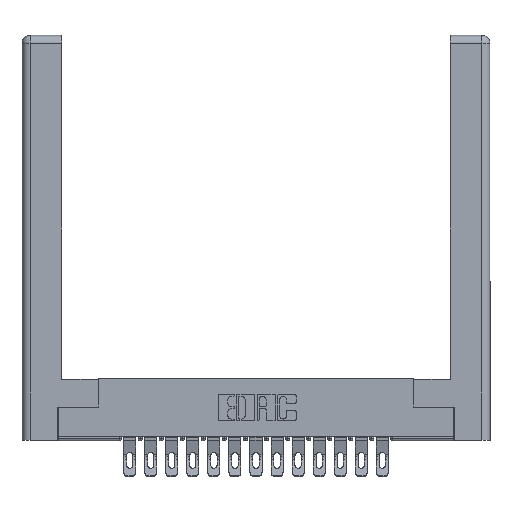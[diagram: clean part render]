
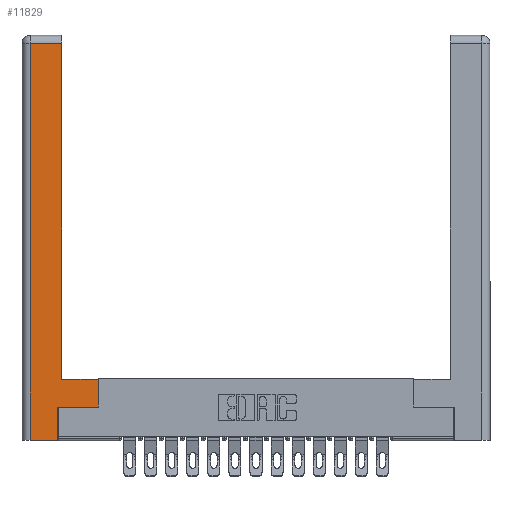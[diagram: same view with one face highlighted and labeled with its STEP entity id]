
A CAD part, top view. The second image highlights one B-rep face of the part: STEP entity #11829.
In plain terms, the highlighted planar face has unit normal (0, 0, 1).
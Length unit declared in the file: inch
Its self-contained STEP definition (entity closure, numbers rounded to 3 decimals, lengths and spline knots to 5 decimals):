
#189 = CARTESIAN_POINT ( 'NONE',  ( 0.265, 0., 0. ) ) ;
#281 = CARTESIAN_POINT ( 'NONE',  ( 0.0615, 2.94, 0. ) ) ;
#295 = PLANE ( 'NONE',  #5100 ) ;
#472 = EDGE_CURVE ( 'NONE', #750, #2969, #9812, .T. ) ;
#750 = VERTEX_POINT ( 'NONE', #14348 ) ;
#1645 = EDGE_CURVE ( 'NONE', #14276, #2510, #8783, .T. ) ;
#2114 = EDGE_CURVE ( 'NONE', #15263, #13758, #15325, .T. ) ;
#2134 = CARTESIAN_POINT ( 'NONE',  ( 0., 0., 0. ) ) ;
#2287 = DIRECTION ( 'NONE',  ( 0., 1., 0. ) ) ;
#2510 = VERTEX_POINT ( 'NONE', #15533 ) ;
#2518 = ORIENTED_EDGE ( 'NONE', *, *, #9903, .T. ) ;
#2969 = VERTEX_POINT ( 'NONE', #12565 ) ;
#3335 = CARTESIAN_POINT ( 'NONE',  ( 0.265, 0., 0. ) ) ;
#3421 = VERTEX_POINT ( 'NONE', #3335 ) ;
#4067 = VECTOR ( 'NONE', #12046, 39.37008 ) ;
#4796 = DIRECTION ( 'NONE',  ( 1., 0., 0. ) ) ;
#5100 = AXIS2_PLACEMENT_3D ( 'NONE', #2134, #5184, #18089 ) ;
#5184 = DIRECTION ( 'NONE',  ( 0., 0., -1. ) ) ;
#5194 = EDGE_CURVE ( 'NONE', #3421, #750, #15138, .T. ) ;
#5506 = ORIENTED_EDGE ( 'NONE', *, *, #1645, .T. ) ;
#6269 = ORIENTED_EDGE ( 'NONE', *, *, #10706, .T. ) ;
#6357 = ORIENTED_EDGE ( 'NONE', *, *, #2114, .T. ) ;
#6869 = EDGE_LOOP ( 'NONE', ( #6269, #2518, #5506, #11358, #15445, #8686, #7670, #6357 ) ) ;
#7189 = LINE ( 'NONE', #281, #16055 ) ;
#7333 = CARTESIAN_POINT ( 'NONE',  ( 0.0615, 2.94, 0. ) ) ;
#7462 = CARTESIAN_POINT ( 'NONE',  ( 0.0615, 0., 0. ) ) ;
#7670 = ORIENTED_EDGE ( 'NONE', *, *, #14121, .T. ) ;
#8174 = CARTESIAN_POINT ( 'NONE',  ( 0.265, 0.245, 0. ) ) ;
#8254 = VECTOR ( 'NONE', #20691, 39.37008 ) ;
#8686 = ORIENTED_EDGE ( 'NONE', *, *, #472, .T. ) ;
#8689 = DIRECTION ( 'NONE',  ( 0., 1., 0. ) ) ;
#8783 = LINE ( 'NONE', #7462, #8254 ) ;
#9812 = LINE ( 'NONE', #12675, #17861 ) ;
#9903 = EDGE_CURVE ( 'NONE', #17333, #14276, #7189, .T. ) ;
#9908 = DIRECTION ( 'NONE',  ( -1., 0., 0. ) ) ;
#9956 = FACE_OUTER_BOUND ( 'NONE', #6869, .T. ) ;
#10320 = EDGE_CURVE ( 'NONE', #2510, #3421, #18059, .T. ) ;
#10481 = VECTOR ( 'NONE', #2287, 39.37008 ) ;
#10706 = EDGE_CURVE ( 'NONE', #13758, #17333, #19535, .T. ) ;
#10826 = CARTESIAN_POINT ( 'NONE',  ( 0.565, 0.45, 0. ) ) ;
#10853 = CARTESIAN_POINT ( 'NONE',  ( 0.295, 2.94, 0. ) ) ;
#10913 = CARTESIAN_POINT ( 'NONE',  ( 0.295, 0.45, 0. ) ) ;
#11358 = ORIENTED_EDGE ( 'NONE', *, *, #10320, .T. ) ;
#11763 = DIRECTION ( 'NONE',  ( -1., 0., 0. ) ) ;
#11829 = ADVANCED_FACE ( 'NONE', ( #9956 ), #295, .F. ) ;
#12046 = DIRECTION ( 'NONE',  ( 0., 1., 0. ) ) ;
#12565 = CARTESIAN_POINT ( 'NONE',  ( 0.565, 0.245, 0. ) ) ;
#12675 = CARTESIAN_POINT ( 'NONE',  ( 0.565, 0.245, 0. ) ) ;
#13100 = CARTESIAN_POINT ( 'NONE',  ( 0.295, 0.45, 0. ) ) ;
#13592 = CARTESIAN_POINT ( 'NONE',  ( 0.565, 0.45, 0. ) ) ;
#13758 = VERTEX_POINT ( 'NONE', #10913 ) ;
#13811 = VECTOR ( 'NONE', #4796, 39.37008 ) ;
#14121 = EDGE_CURVE ( 'NONE', #2969, #15263, #14898, .T. ) ;
#14276 = VERTEX_POINT ( 'NONE', #7333 ) ;
#14348 = CARTESIAN_POINT ( 'NONE',  ( 0.265, 0.245, 0. ) ) ;
#14898 = LINE ( 'NONE', #13592, #4067 ) ;
#15138 = LINE ( 'NONE', #8174, #16646 ) ;
#15263 = VERTEX_POINT ( 'NONE', #10826 ) ;
#15325 = LINE ( 'NONE', #13100, #16849 ) ;
#15445 = ORIENTED_EDGE ( 'NONE', *, *, #5194, .T. ) ;
#15533 = CARTESIAN_POINT ( 'NONE',  ( 0.0615, 0., 0. ) ) ;
#16055 = VECTOR ( 'NONE', #11763, 39.37008 ) ;
#16646 = VECTOR ( 'NONE', #8689, 39.37008 ) ;
#16849 = VECTOR ( 'NONE', #9908, 39.37008 ) ;
#17256 = DIRECTION ( 'NONE',  ( 1., 0., 0. ) ) ;
#17333 = VERTEX_POINT ( 'NONE', #10853 ) ;
#17861 = VECTOR ( 'NONE', #17256, 39.37008 ) ;
#18059 = LINE ( 'NONE', #189, #13811 ) ;
#18089 = DIRECTION ( 'NONE',  ( -1., 0., 0. ) ) ;
#18524 = CARTESIAN_POINT ( 'NONE',  ( 0.295, 3., 0. ) ) ;
#19535 = LINE ( 'NONE', #18524, #10481 ) ;
#20691 = DIRECTION ( 'NONE',  ( 0., -1., 0. ) ) ;
